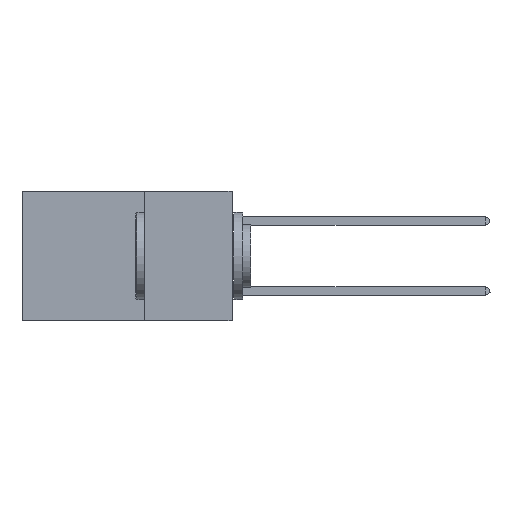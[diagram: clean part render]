
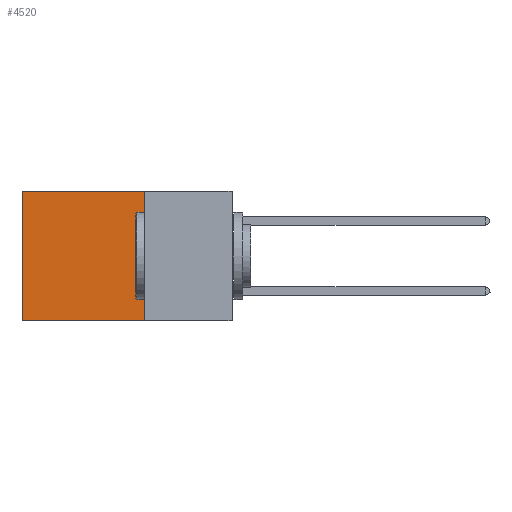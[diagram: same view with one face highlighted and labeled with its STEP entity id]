
A CAD part, left-side view. The second image highlights one B-rep face of the part: STEP entity #4520.
In plain terms, the highlighted planar face has unit normal (-1, 0, 0).
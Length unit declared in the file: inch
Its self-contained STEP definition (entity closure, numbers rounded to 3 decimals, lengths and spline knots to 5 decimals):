
#660 = CARTESIAN_POINT ( 'NONE',  ( 0.2875, 0.25, -0.37 ) ) ;
#1087 = ORIENTED_EDGE ( 'NONE', *, *, #1207, .T. ) ;
#1207 = EDGE_CURVE ( 'NONE', #3014, #15820, #4496, .T. ) ;
#1732 = VERTEX_POINT ( 'NONE', #660 ) ;
#1986 = VERTEX_POINT ( 'NONE', #12072 ) ;
#3014 = VERTEX_POINT ( 'NONE', #13453 ) ;
#3542 = LINE ( 'NONE', #13687, #5268 ) ;
#3898 = EDGE_CURVE ( 'NONE', #15820, #1986, #3542, .T. ) ;
#4496 = LINE ( 'NONE', #13735, #6903 ) ;
#4520 = ADVANCED_FACE ( 'NONE', ( #11505 ), #16851, .F. ) ;
#4619 = DIRECTION ( 'NONE',  ( 1., 0., 0. ) ) ;
#5268 = VECTOR ( 'NONE', #10714, 39.37008 ) ;
#5333 = CARTESIAN_POINT ( 'NONE',  ( 0.2875, 0.25, -0.37 ) ) ;
#6064 = AXIS2_PLACEMENT_3D ( 'NONE', #14212, #4619, #14280 ) ;
#6903 = VECTOR ( 'NONE', #12426, 39.37008 ) ;
#7708 = EDGE_CURVE ( 'NONE', #3014, #1732, #17045, .T. ) ;
#7804 = VECTOR ( 'NONE', #15352, 39.37008 ) ;
#8739 = ORIENTED_EDGE ( 'NONE', *, *, #13363, .F. ) ;
#8866 = CARTESIAN_POINT ( 'NONE',  ( 0.2875, 0.6, 0. ) ) ;
#10376 = LINE ( 'NONE', #5333, #15797 ) ;
#10714 = DIRECTION ( 'NONE',  ( 0., 0., -1. ) ) ;
#11505 = FACE_OUTER_BOUND ( 'NONE', #15461, .T. ) ;
#12003 = ORIENTED_EDGE ( 'NONE', *, *, #7708, .F. ) ;
#12072 = CARTESIAN_POINT ( 'NONE',  ( 0.2875, 0.6, -0.37 ) ) ;
#12400 = ORIENTED_EDGE ( 'NONE', *, *, #3898, .T. ) ;
#12426 = DIRECTION ( 'NONE',  ( 0., 1., 0. ) ) ;
#13363 = EDGE_CURVE ( 'NONE', #1732, #1986, #10376, .T. ) ;
#13453 = CARTESIAN_POINT ( 'NONE',  ( 0.2875, 0.25, 0. ) ) ;
#13687 = CARTESIAN_POINT ( 'NONE',  ( 0.2875, 0.6, 0. ) ) ;
#13735 = CARTESIAN_POINT ( 'NONE',  ( 0.2875, 0.25, 0. ) ) ;
#13938 = CARTESIAN_POINT ( 'NONE',  ( 0.2875, 0.25, 0. ) ) ;
#14212 = CARTESIAN_POINT ( 'NONE',  ( 0.2875, 0.25, 0. ) ) ;
#14280 = DIRECTION ( 'NONE',  ( 0., 0., -1. ) ) ;
#15352 = DIRECTION ( 'NONE',  ( 0., 0., -1. ) ) ;
#15461 = EDGE_LOOP ( 'NONE', ( #12400, #8739, #12003, #1087 ) ) ;
#15797 = VECTOR ( 'NONE', #16321, 39.37008 ) ;
#15820 = VERTEX_POINT ( 'NONE', #8866 ) ;
#16321 = DIRECTION ( 'NONE',  ( 0., 1., 0. ) ) ;
#16851 = PLANE ( 'NONE',  #6064 ) ;
#17045 = LINE ( 'NONE', #13938, #7804 ) ;
